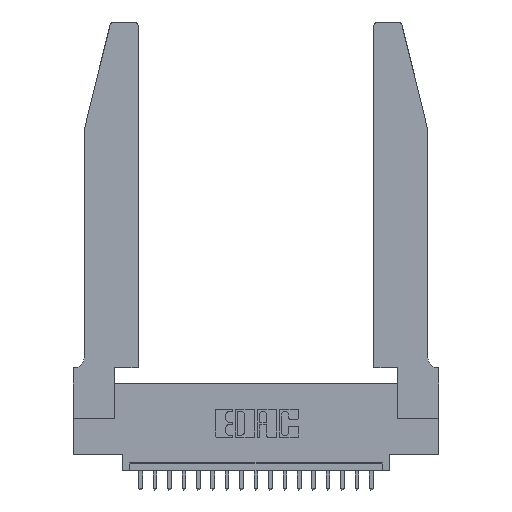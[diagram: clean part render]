
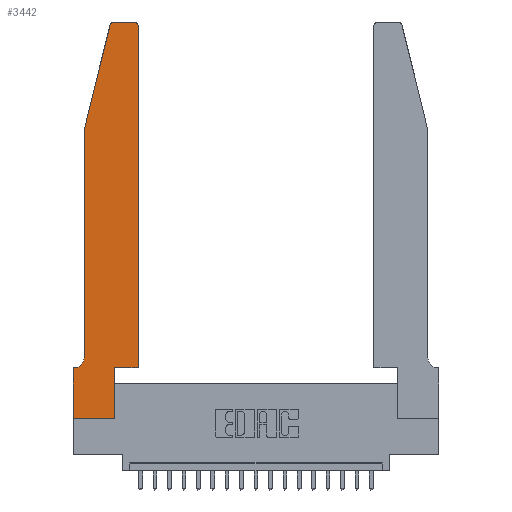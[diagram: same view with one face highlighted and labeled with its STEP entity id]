
A CAD part, top view. The second image highlights one B-rep face of the part: STEP entity #3442.
In plain terms, the highlighted planar face has unit normal (0, 0, 1).
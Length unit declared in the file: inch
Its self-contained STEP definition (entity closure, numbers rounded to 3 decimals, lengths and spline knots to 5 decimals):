
#5 = LINE ( 'NONE', #8894, #2788 ) ;
#167 = VERTEX_POINT ( 'NONE', #6508 ) ;
#568 = CARTESIAN_POINT ( 'NONE',  ( 0., 0., 0.37 ) ) ;
#828 = CARTESIAN_POINT ( 'NONE',  ( 0.4205, 2.72, 0.37 ) ) ;
#1125 = VERTEX_POINT ( 'NONE', #11429 ) ;
#1523 = AXIS2_PLACEMENT_3D ( 'NONE', #828, #9143, #17040 ) ;
#1632 = LINE ( 'NONE', #13784, #10556 ) ;
#1858 = CARTESIAN_POINT ( 'NONE',  ( 0., 0.35, 0.37 ) ) ;
#1996 = PLANE ( 'NONE',  #13409 ) ;
#2138 = EDGE_CURVE ( 'NONE', #19423, #19736, #2546, .T. ) ;
#2427 = DIRECTION ( 'NONE',  ( 0., -1., 0. ) ) ;
#2546 = CIRCLE ( 'NONE', #1523, 0.03 ) ;
#2577 = DIRECTION ( 'NONE',  ( 0., 0., 1. ) ) ;
#2704 = DIRECTION ( 'NONE',  ( -1., 0., 0. ) ) ;
#2719 = DIRECTION ( 'NONE',  ( 1., 0., 0. ) ) ;
#2728 = CARTESIAN_POINT ( 'NONE',  ( 0.2865, 0., 0.37 ) ) ;
#2746 = VERTEX_POINT ( 'NONE', #17497 ) ;
#2788 = VECTOR ( 'NONE', #7403, 39.37008 ) ;
#2847 = LINE ( 'NONE', #11369, #19927 ) ;
#3041 = VECTOR ( 'NONE', #8022, 39.37008 ) ;
#3315 = VERTEX_POINT ( 'NONE', #3354 ) ;
#3354 = CARTESIAN_POINT ( 'NONE',  ( 0.284, 2.75, 0.37 ) ) ;
#3442 = ADVANCED_FACE ( 'NONE', ( #11147 ), #1996, .T. ) ;
#3561 = CARTESIAN_POINT ( 'NONE',  ( 0.0755, 2., 0.37 ) ) ;
#3691 = ORIENTED_EDGE ( 'NONE', *, *, #12544, .T. ) ;
#3790 = DIRECTION ( 'NONE',  ( 1., 0., 0. ) ) ;
#3820 = DIRECTION ( 'NONE',  ( -1., 0., 0. ) ) ;
#4193 = LINE ( 'NONE', #7630, #7502 ) ;
#4408 = VECTOR ( 'NONE', #6401, 39.37008 ) ;
#5153 = EDGE_CURVE ( 'NONE', #167, #17772, #8288, .T. ) ;
#5185 = DIRECTION ( 'NONE',  ( 0., -1., 0. ) ) ;
#5390 = CARTESIAN_POINT ( 'NONE',  ( 0.4505, 0.35, 0.37 ) ) ;
#5711 = EDGE_CURVE ( 'NONE', #15102, #167, #1632, .T. ) ;
#6401 = DIRECTION ( 'NONE',  ( 0., 1., 0. ) ) ;
#6470 = DIRECTION ( 'NONE',  ( 1., 0., 0. ) ) ;
#6508 = CARTESIAN_POINT ( 'NONE',  ( 0., 0., 0.37 ) ) ;
#6513 = CARTESIAN_POINT ( 'NONE',  ( 0.0755, 0.42, 0.37 ) ) ;
#6641 = CARTESIAN_POINT ( 'NONE',  ( 0.4205, 2.75, 0.37 ) ) ;
#7035 = CIRCLE ( 'NONE', #7849, 0.07 ) ;
#7273 = VECTOR ( 'NONE', #8747, 39.37008 ) ;
#7403 = DIRECTION ( 'NONE',  ( -0.239, -0.971, 0. ) ) ;
#7502 = VECTOR ( 'NONE', #2704, 39.37008 ) ;
#7630 = CARTESIAN_POINT ( 'NONE',  ( 0.0755, 0.35, 0.37 ) ) ;
#7849 = AXIS2_PLACEMENT_3D ( 'NONE', #13569, #16831, #3820 ) ;
#7918 = ORIENTED_EDGE ( 'NONE', *, *, #2138, .T. ) ;
#8022 = DIRECTION ( 'NONE',  ( 0., 1., 0. ) ) ;
#8135 = EDGE_CURVE ( 'NONE', #15833, #10105, #7035, .T. ) ;
#8288 = LINE ( 'NONE', #568, #7273 ) ;
#8747 = DIRECTION ( 'NONE',  ( 1., 0., 0. ) ) ;
#8894 = CARTESIAN_POINT ( 'NONE',  ( 0.0755, 2., 0.37 ) ) ;
#9143 = DIRECTION ( 'NONE',  ( 0., 0., 1. ) ) ;
#9162 = AXIS2_PLACEMENT_3D ( 'NONE', #19018, #2577, #2719 ) ;
#9867 = ORIENTED_EDGE ( 'NONE', *, *, #5153, .T. ) ;
#10105 = VERTEX_POINT ( 'NONE', #13112 ) ;
#10190 = VECTOR ( 'NONE', #5185, 39.37008 ) ;
#10264 = DIRECTION ( 'NONE',  ( 0., 0., 1. ) ) ;
#10311 = ORIENTED_EDGE ( 'NONE', *, *, #10708, .T. ) ;
#10556 = VECTOR ( 'NONE', #2427, 39.37008 ) ;
#10678 = LINE ( 'NONE', #20611, #3041 ) ;
#10691 = CARTESIAN_POINT ( 'NONE',  ( 0.4505, 2.72, 0.37 ) ) ;
#10703 = ORIENTED_EDGE ( 'NONE', *, *, #14527, .T. ) ;
#10708 = EDGE_CURVE ( 'NONE', #17772, #12417, #13072, .T. ) ;
#10835 = EDGE_CURVE ( 'NONE', #12417, #11354, #2847, .T. ) ;
#11047 = CARTESIAN_POINT ( 'NONE',  ( 0.2605, 2.75, 0.37 ) ) ;
#11147 = FACE_OUTER_BOUND ( 'NONE', #11568, .T. ) ;
#11354 = VERTEX_POINT ( 'NONE', #5390 ) ;
#11369 = CARTESIAN_POINT ( 'NONE',  ( 0.4505, 0.35, 0.37 ) ) ;
#11371 = CARTESIAN_POINT ( 'NONE',  ( 0.2865, 0.35, 0.37 ) ) ;
#11429 = CARTESIAN_POINT ( 'NONE',  ( 0.25487, 2.72718, 0.37 ) ) ;
#11568 = EDGE_LOOP ( 'NONE', ( #17896, #20496, #15937, #3691, #17354, #10703, #14004, #9867, #10311, #12596, #15896, #7918 ) ) ;
#12417 = VERTEX_POINT ( 'NONE', #14740 ) ;
#12544 = EDGE_CURVE ( 'NONE', #2746, #15833, #13232, .T. ) ;
#12596 = ORIENTED_EDGE ( 'NONE', *, *, #10835, .T. ) ;
#12983 = DIRECTION ( 'NONE',  ( -1., 0., 0. ) ) ;
#13072 = LINE ( 'NONE', #11371, #4408 ) ;
#13112 = CARTESIAN_POINT ( 'NONE',  ( 0.0055, 0.35, 0.37 ) ) ;
#13232 = LINE ( 'NONE', #3561, #10190 ) ;
#13409 = AXIS2_PLACEMENT_3D ( 'NONE', #1858, #10264, #3790 ) ;
#13569 = CARTESIAN_POINT ( 'NONE',  ( 0.0055, 0.42, 0.37 ) ) ;
#13784 = CARTESIAN_POINT ( 'NONE',  ( 0., 0., 0.37 ) ) ;
#14004 = ORIENTED_EDGE ( 'NONE', *, *, #5711, .T. ) ;
#14092 = EDGE_CURVE ( 'NONE', #3315, #1125, #19205, .T. ) ;
#14527 = EDGE_CURVE ( 'NONE', #10105, #15102, #4193, .T. ) ;
#14740 = CARTESIAN_POINT ( 'NONE',  ( 0.2865, 0.35, 0.37 ) ) ;
#14804 = VECTOR ( 'NONE', #12983, 39.37008 ) ;
#15102 = VERTEX_POINT ( 'NONE', #15789 ) ;
#15318 = LINE ( 'NONE', #11047, #14804 ) ;
#15789 = CARTESIAN_POINT ( 'NONE',  ( 0., 0.35, 0.37 ) ) ;
#15833 = VERTEX_POINT ( 'NONE', #6513 ) ;
#15896 = ORIENTED_EDGE ( 'NONE', *, *, #17151, .T. ) ;
#15937 = ORIENTED_EDGE ( 'NONE', *, *, #17073, .T. ) ;
#16831 = DIRECTION ( 'NONE',  ( 0., 0., -1. ) ) ;
#17040 = DIRECTION ( 'NONE',  ( 1., 0., 0. ) ) ;
#17073 = EDGE_CURVE ( 'NONE', #1125, #2746, #5, .T. ) ;
#17151 = EDGE_CURVE ( 'NONE', #11354, #19423, #10678, .T. ) ;
#17354 = ORIENTED_EDGE ( 'NONE', *, *, #8135, .T. ) ;
#17497 = CARTESIAN_POINT ( 'NONE',  ( 0.0755, 2., 0.37 ) ) ;
#17772 = VERTEX_POINT ( 'NONE', #2728 ) ;
#17896 = ORIENTED_EDGE ( 'NONE', *, *, #20944, .T. ) ;
#19018 = CARTESIAN_POINT ( 'NONE',  ( 0.284, 2.72, 0.37 ) ) ;
#19205 = CIRCLE ( 'NONE', #9162, 0.03 ) ;
#19423 = VERTEX_POINT ( 'NONE', #10691 ) ;
#19736 = VERTEX_POINT ( 'NONE', #6641 ) ;
#19927 = VECTOR ( 'NONE', #6470, 39.37008 ) ;
#20496 = ORIENTED_EDGE ( 'NONE', *, *, #14092, .T. ) ;
#20611 = CARTESIAN_POINT ( 'NONE',  ( 0.4505, 0.35, 0.37 ) ) ;
#20944 = EDGE_CURVE ( 'NONE', #19736, #3315, #15318, .T. ) ;
